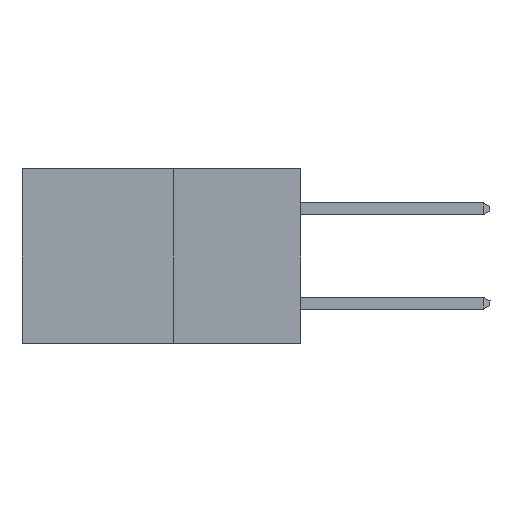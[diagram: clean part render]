
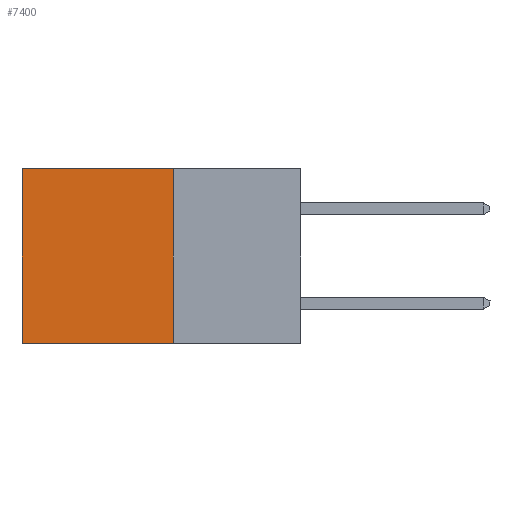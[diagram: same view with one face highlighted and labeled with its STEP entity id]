
A CAD part, left-side view. The second image highlights one B-rep face of the part: STEP entity #7400.
In plain terms, the highlighted planar face has unit normal (-1, 0, 0).
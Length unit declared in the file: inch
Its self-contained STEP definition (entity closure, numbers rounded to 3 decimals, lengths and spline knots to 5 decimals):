
#3578 = DIRECTION ( 'NONE',  ( 0., 0., -1. ) ) ;
#4151 = CARTESIAN_POINT ( 'NONE',  ( 0.277, 0.27, -0.37 ) ) ;
#4932 = LINE ( 'NONE', #8964, #5729 ) ;
#5729 = VECTOR ( 'NONE', #21250, 39.37008 ) ;
#6150 = FACE_OUTER_BOUND ( 'NONE', #7846, .T. ) ;
#6948 = EDGE_CURVE ( 'NONE', #12542, #27879, #4932, .T. ) ;
#7019 = VECTOR ( 'NONE', #3578, 39.37008 ) ;
#7400 = ADVANCED_FACE ( 'NONE', ( #6150 ), #10423, .F. ) ;
#7798 = LINE ( 'NONE', #16205, #7019 ) ;
#7846 = EDGE_LOOP ( 'NONE', ( #16871, #25918, #20847, #13933 ) ) ;
#8964 = CARTESIAN_POINT ( 'NONE',  ( 0.277, 0.27, 0. ) ) ;
#10423 = PLANE ( 'NONE',  #30630 ) ;
#10468 = DIRECTION ( 'NONE',  ( 0., 0., -1. ) ) ;
#10720 = VECTOR ( 'NONE', #31980, 39.37008 ) ;
#11494 = VERTEX_POINT ( 'NONE', #4151 ) ;
#12214 = EDGE_CURVE ( 'NONE', #11494, #21197, #23364, .T. ) ;
#12542 = VERTEX_POINT ( 'NONE', #25538 ) ;
#12712 = CARTESIAN_POINT ( 'NONE',  ( 0.277, 0.27, -0.37 ) ) ;
#13125 = CARTESIAN_POINT ( 'NONE',  ( 0.277, 0.59, 0. ) ) ;
#13933 = ORIENTED_EDGE ( 'NONE', *, *, #6948, .T. ) ;
#14384 = EDGE_CURVE ( 'NONE', #12542, #11494, #14555, .T. ) ;
#14555 = LINE ( 'NONE', #30636, #19690 ) ;
#16205 = CARTESIAN_POINT ( 'NONE',  ( 0.277, 0.59, -0.37 ) ) ;
#16206 = DIRECTION ( 'NONE',  ( 1., 0., 0. ) ) ;
#16871 = ORIENTED_EDGE ( 'NONE', *, *, #26627, .T. ) ;
#19690 = VECTOR ( 'NONE', #10468, 39.37008 ) ;
#20847 = ORIENTED_EDGE ( 'NONE', *, *, #14384, .F. ) ;
#21197 = VERTEX_POINT ( 'NONE', #31766 ) ;
#21250 = DIRECTION ( 'NONE',  ( 0., 1., 0. ) ) ;
#23364 = LINE ( 'NONE', #26979, #10720 ) ;
#25538 = CARTESIAN_POINT ( 'NONE',  ( 0.277, 0.27, 0. ) ) ;
#25918 = ORIENTED_EDGE ( 'NONE', *, *, #12214, .F. ) ;
#26095 = DIRECTION ( 'NONE',  ( 0., 0., -1. ) ) ;
#26627 = EDGE_CURVE ( 'NONE', #27879, #21197, #7798, .T. ) ;
#26979 = CARTESIAN_POINT ( 'NONE',  ( 0.277, 0.27, -0.37 ) ) ;
#27879 = VERTEX_POINT ( 'NONE', #13125 ) ;
#30630 = AXIS2_PLACEMENT_3D ( 'NONE', #12712, #16206, #26095 ) ;
#30636 = CARTESIAN_POINT ( 'NONE',  ( 0.277, 0.27, -0.37 ) ) ;
#31766 = CARTESIAN_POINT ( 'NONE',  ( 0.277, 0.59, -0.37 ) ) ;
#31980 = DIRECTION ( 'NONE',  ( 0., 1., 0. ) ) ;
